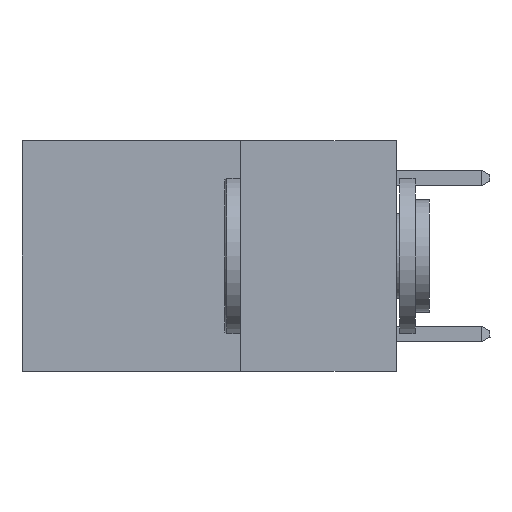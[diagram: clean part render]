
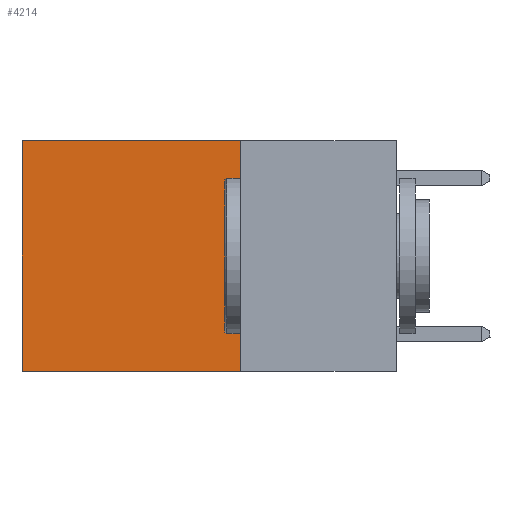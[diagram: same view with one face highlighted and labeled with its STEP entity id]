
A CAD part, left-side view. The second image highlights one B-rep face of the part: STEP entity #4214.
In plain terms, the highlighted planar face has unit normal (-1, 0, 0).
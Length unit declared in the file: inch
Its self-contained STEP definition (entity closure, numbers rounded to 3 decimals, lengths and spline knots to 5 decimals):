
#1192 = LINE ( 'NONE', #4778, #11963 ) ;
#1222 = VERTEX_POINT ( 'NONE', #6545 ) ;
#1369 = LINE ( 'NONE', #12022, #12869 ) ;
#1520 = EDGE_CURVE ( 'NONE', #1222, #13268, #1369, .T. ) ;
#1791 = CARTESIAN_POINT ( 'NONE',  ( 0.2625, 0.6, 0. ) ) ;
#1892 = DIRECTION ( 'NONE',  ( 1., 0., 0. ) ) ;
#2117 = ORIENTED_EDGE ( 'NONE', *, *, #9853, .F. ) ;
#2587 = LINE ( 'NONE', #11668, #6473 ) ;
#3395 = ORIENTED_EDGE ( 'NONE', *, *, #5278, .F. ) ;
#4152 = AXIS2_PLACEMENT_3D ( 'NONE', #13504, #1892, #9779 ) ;
#4214 = ADVANCED_FACE ( 'NONE', ( #5367 ), #10002, .F. ) ;
#4778 = CARTESIAN_POINT ( 'NONE',  ( 0.2625, 0.25, -0.37 ) ) ;
#4818 = DIRECTION ( 'NONE',  ( 0., 0., -1. ) ) ;
#5278 = EDGE_CURVE ( 'NONE', #12241, #14587, #1192, .T. ) ;
#5367 = FACE_OUTER_BOUND ( 'NONE', #7754, .T. ) ;
#5466 = ORIENTED_EDGE ( 'NONE', *, *, #1520, .T. ) ;
#5593 = CARTESIAN_POINT ( 'NONE',  ( 0.2625, 0.25, -0.37 ) ) ;
#5836 = CARTESIAN_POINT ( 'NONE',  ( 0.2625, 0.6, -0.37 ) ) ;
#6458 = DIRECTION ( 'NONE',  ( 0., 0., -1. ) ) ;
#6473 = VECTOR ( 'NONE', #4818, 39.37008 ) ;
#6545 = CARTESIAN_POINT ( 'NONE',  ( 0.2625, 0.25, 0. ) ) ;
#7754 = EDGE_LOOP ( 'NONE', ( #12549, #3395, #2117, #5466 ) ) ;
#8220 = DIRECTION ( 'NONE',  ( 0., 1., 0. ) ) ;
#9433 = DIRECTION ( 'NONE',  ( 0., 1., 0. ) ) ;
#9779 = DIRECTION ( 'NONE',  ( 0., 0., -1. ) ) ;
#9853 = EDGE_CURVE ( 'NONE', #1222, #12241, #2587, .T. ) ;
#10002 = PLANE ( 'NONE',  #4152 ) ;
#10085 = CARTESIAN_POINT ( 'NONE',  ( 0.2625, 0.6, 0. ) ) ;
#10890 = LINE ( 'NONE', #1791, #14790 ) ;
#11668 = CARTESIAN_POINT ( 'NONE',  ( 0.2625, 0.25, 0. ) ) ;
#11963 = VECTOR ( 'NONE', #9433, 39.37008 ) ;
#12022 = CARTESIAN_POINT ( 'NONE',  ( 0.2625, 0.25, 0. ) ) ;
#12241 = VERTEX_POINT ( 'NONE', #5593 ) ;
#12549 = ORIENTED_EDGE ( 'NONE', *, *, #13994, .T. ) ;
#12869 = VECTOR ( 'NONE', #8220, 39.37008 ) ;
#13268 = VERTEX_POINT ( 'NONE', #10085 ) ;
#13504 = CARTESIAN_POINT ( 'NONE',  ( 0.2625, 0.25, 0. ) ) ;
#13994 = EDGE_CURVE ( 'NONE', #13268, #14587, #10890, .T. ) ;
#14587 = VERTEX_POINT ( 'NONE', #5836 ) ;
#14790 = VECTOR ( 'NONE', #6458, 39.37008 ) ;
